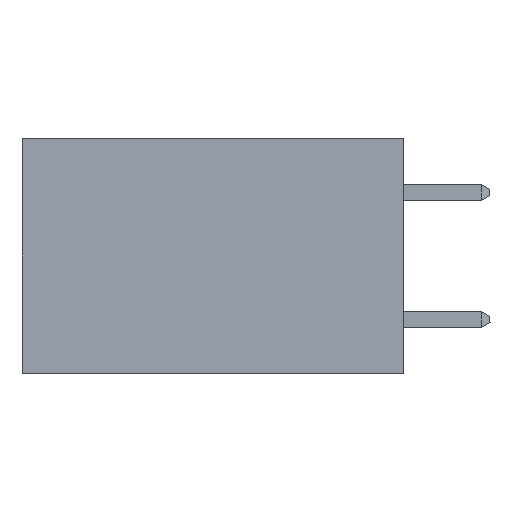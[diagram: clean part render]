
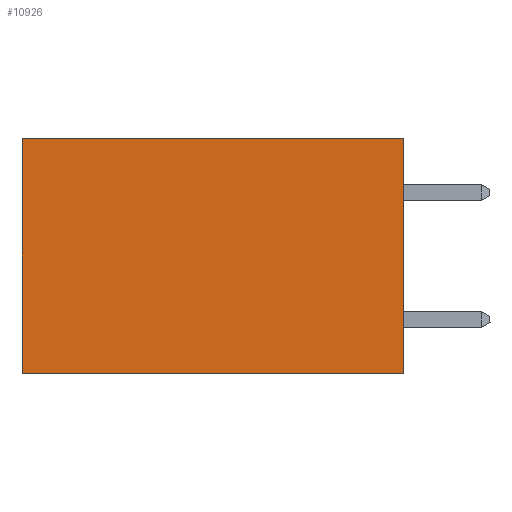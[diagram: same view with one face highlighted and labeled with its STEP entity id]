
A CAD part, left-side view. The second image highlights one B-rep face of the part: STEP entity #10926.
In plain terms, the highlighted planar face has unit normal (-1, 0, 0).
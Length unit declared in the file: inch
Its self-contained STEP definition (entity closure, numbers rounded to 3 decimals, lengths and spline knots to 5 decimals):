
#2465 = VECTOR ( 'NONE', #19235, 39.37008 ) ;
#3031 = ORIENTED_EDGE ( 'NONE', *, *, #20049, .F. ) ;
#4644 = AXIS2_PLACEMENT_3D ( 'NONE', #6829, #24020, #17713 ) ;
#5430 = ORIENTED_EDGE ( 'NONE', *, *, #18389, .F. ) ;
#6829 = CARTESIAN_POINT ( 'NONE',  ( 0.2875, 0., 0. ) ) ;
#7722 = LINE ( 'NONE', #19967, #22738 ) ;
#7741 = EDGE_CURVE ( 'NONE', #25246, #25320, #15586, .T. ) ;
#8827 = ORIENTED_EDGE ( 'NONE', *, *, #7741, .T. ) ;
#9872 = CARTESIAN_POINT ( 'NONE',  ( 0.2875, 0.6, 0. ) ) ;
#10700 = PLANE ( 'NONE',  #4644 ) ;
#10926 = ADVANCED_FACE ( 'NONE', ( #17406 ), #10700, .F. ) ;
#11433 = LINE ( 'NONE', #21378, #2465 ) ;
#12377 = EDGE_CURVE ( 'NONE', #25320, #14392, #13670, .T. ) ;
#13670 = LINE ( 'NONE', #9872, #17027 ) ;
#14392 = VERTEX_POINT ( 'NONE', #27701 ) ;
#14732 = CARTESIAN_POINT ( 'NONE',  ( 0.2875, 0.6, 0. ) ) ;
#15586 = LINE ( 'NONE', #21894, #16259 ) ;
#16259 = VECTOR ( 'NONE', #20858, 39.37008 ) ;
#17027 = VECTOR ( 'NONE', #24890, 39.37008 ) ;
#17406 = FACE_OUTER_BOUND ( 'NONE', #25190, .T. ) ;
#17713 = DIRECTION ( 'NONE',  ( 0., 0., -1. ) ) ;
#17819 = DIRECTION ( 'NONE',  ( 0., 1., 0. ) ) ;
#18162 = ORIENTED_EDGE ( 'NONE', *, *, #12377, .T. ) ;
#18389 = EDGE_CURVE ( 'NONE', #25234, #14392, #7722, .T. ) ;
#19235 = DIRECTION ( 'NONE',  ( 0., 0., -1. ) ) ;
#19967 = CARTESIAN_POINT ( 'NONE',  ( 0.2875, 0., -0.37 ) ) ;
#20049 = EDGE_CURVE ( 'NONE', #25246, #25234, #11433, .T. ) ;
#20858 = DIRECTION ( 'NONE',  ( 0., 1., 0. ) ) ;
#21013 = CARTESIAN_POINT ( 'NONE',  ( 0.2875, 0., 0. ) ) ;
#21378 = CARTESIAN_POINT ( 'NONE',  ( 0.2875, 0., 0. ) ) ;
#21894 = CARTESIAN_POINT ( 'NONE',  ( 0.2875, 0., 0. ) ) ;
#22738 = VECTOR ( 'NONE', #17819, 39.37008 ) ;
#24020 = DIRECTION ( 'NONE',  ( 1., 0., 0. ) ) ;
#24890 = DIRECTION ( 'NONE',  ( 0., 0., -1. ) ) ;
#25190 = EDGE_LOOP ( 'NONE', ( #18162, #5430, #3031, #8827 ) ) ;
#25234 = VERTEX_POINT ( 'NONE', #27152 ) ;
#25246 = VERTEX_POINT ( 'NONE', #21013 ) ;
#25320 = VERTEX_POINT ( 'NONE', #14732 ) ;
#27152 = CARTESIAN_POINT ( 'NONE',  ( 0.2875, 0., -0.37 ) ) ;
#27701 = CARTESIAN_POINT ( 'NONE',  ( 0.2875, 0.6, -0.37 ) ) ;
